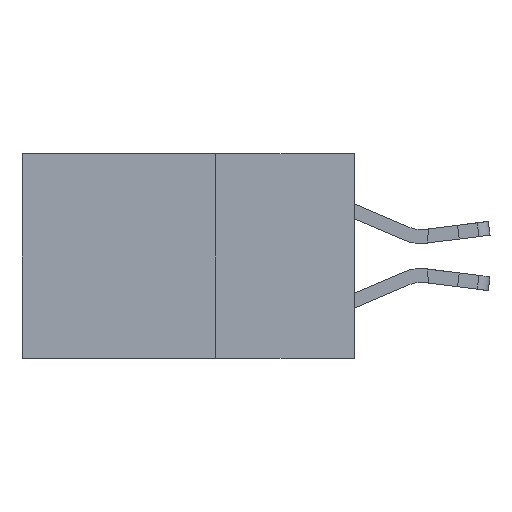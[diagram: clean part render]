
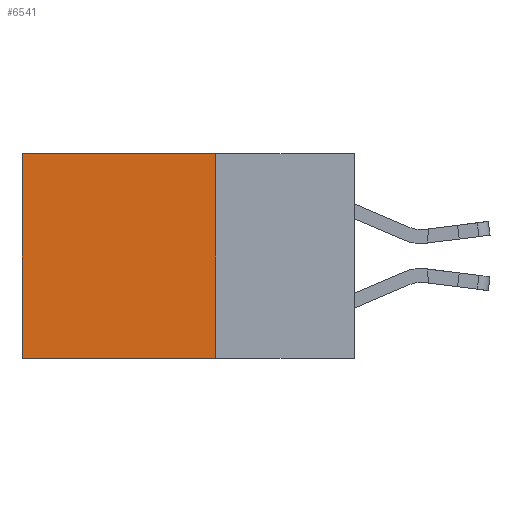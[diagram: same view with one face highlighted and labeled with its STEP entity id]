
A CAD part, left-side view. The second image highlights one B-rep face of the part: STEP entity #6541.
In plain terms, the highlighted planar face has unit normal (-1, 0, 0).
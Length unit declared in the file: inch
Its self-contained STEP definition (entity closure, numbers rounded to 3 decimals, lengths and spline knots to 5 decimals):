
#212 = ORIENTED_EDGE ( 'NONE', *, *, #3656, .T. ) ;
#1996 = VERTEX_POINT ( 'NONE', #8809 ) ;
#2030 = EDGE_LOOP ( 'NONE', ( #212, #3511, #2536, #7119 ) ) ;
#2207 = VERTEX_POINT ( 'NONE', #7570 ) ;
#2536 = ORIENTED_EDGE ( 'NONE', *, *, #11492, .F. ) ;
#2866 = EDGE_CURVE ( 'NONE', #1996, #11541, #9120, .T. ) ;
#3240 = DIRECTION ( 'NONE',  ( 0., 0., -1. ) ) ;
#3347 = AXIS2_PLACEMENT_3D ( 'NONE', #11176, #10229, #4319 ) ;
#3511 = ORIENTED_EDGE ( 'NONE', *, *, #7495, .F. ) ;
#3656 = EDGE_CURVE ( 'NONE', #11541, #2207, #5692, .T. ) ;
#3733 = VECTOR ( 'NONE', #9996, 39.37008 ) ;
#3949 = CARTESIAN_POINT ( 'NONE',  ( 0.2615, 0.25, -0.37 ) ) ;
#4319 = DIRECTION ( 'NONE',  ( 0., 0., -1. ) ) ;
#4448 = FACE_OUTER_BOUND ( 'NONE', #2030, .T. ) ;
#4509 = PLANE ( 'NONE',  #3347 ) ;
#5351 = CARTESIAN_POINT ( 'NONE',  ( 0.2615, 0.25, -0.37 ) ) ;
#5466 = CARTESIAN_POINT ( 'NONE',  ( 0.2615, 0.6, 0. ) ) ;
#5476 = LINE ( 'NONE', #5351, #12079 ) ;
#5692 = LINE ( 'NONE', #8575, #11499 ) ;
#6541 = ADVANCED_FACE ( 'NONE', ( #4448 ), #4509, .F. ) ;
#7119 = ORIENTED_EDGE ( 'NONE', *, *, #2866, .T. ) ;
#7495 = EDGE_CURVE ( 'NONE', #10161, #2207, #5476, .T. ) ;
#7570 = CARTESIAN_POINT ( 'NONE',  ( 0.2615, 0.6, -0.37 ) ) ;
#8041 = LINE ( 'NONE', #11868, #8090 ) ;
#8090 = VECTOR ( 'NONE', #3240, 39.37008 ) ;
#8575 = CARTESIAN_POINT ( 'NONE',  ( 0.2615, 0.6, -0.37 ) ) ;
#8809 = CARTESIAN_POINT ( 'NONE',  ( 0.2615, 0.25, 0. ) ) ;
#9120 = LINE ( 'NONE', #10800, #3733 ) ;
#9996 = DIRECTION ( 'NONE',  ( 0., 1., 0. ) ) ;
#10059 = DIRECTION ( 'NONE',  ( 0., 1., 0. ) ) ;
#10161 = VERTEX_POINT ( 'NONE', #3949 ) ;
#10229 = DIRECTION ( 'NONE',  ( 1., 0., 0. ) ) ;
#10800 = CARTESIAN_POINT ( 'NONE',  ( 0.2615, 0.25, 0. ) ) ;
#11176 = CARTESIAN_POINT ( 'NONE',  ( 0.2615, 0.25, -0.37 ) ) ;
#11492 = EDGE_CURVE ( 'NONE', #1996, #10161, #8041, .T. ) ;
#11499 = VECTOR ( 'NONE', #11529, 39.37008 ) ;
#11529 = DIRECTION ( 'NONE',  ( 0., 0., -1. ) ) ;
#11541 = VERTEX_POINT ( 'NONE', #5466 ) ;
#11868 = CARTESIAN_POINT ( 'NONE',  ( 0.2615, 0.25, -0.37 ) ) ;
#12079 = VECTOR ( 'NONE', #10059, 39.37008 ) ;
